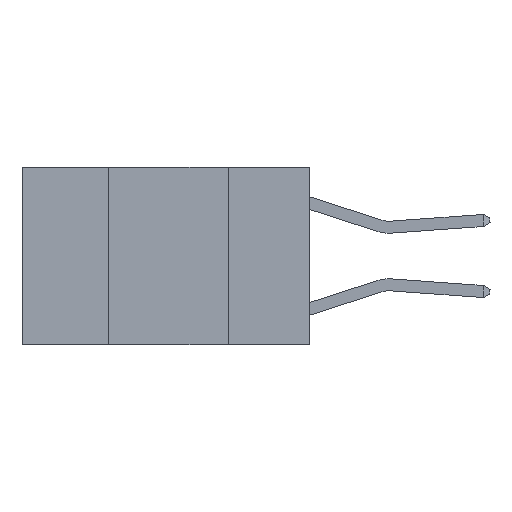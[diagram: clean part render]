
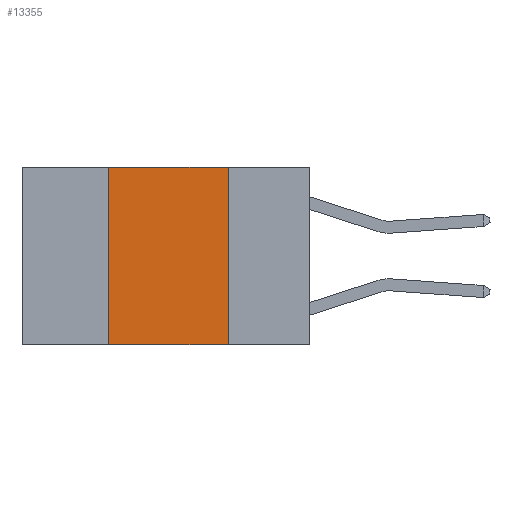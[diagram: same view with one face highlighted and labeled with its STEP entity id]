
A CAD part, left-side view. The second image highlights one B-rep face of the part: STEP entity #13355.
In plain terms, the highlighted planar face has unit normal (-1, 0, 0).
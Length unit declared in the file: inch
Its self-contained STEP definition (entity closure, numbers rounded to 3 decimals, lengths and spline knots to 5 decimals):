
#691 = DIRECTION ( 'NONE',  ( 1., 0., 0. ) ) ;
#2619 = VERTEX_POINT ( 'NONE', #2641 ) ;
#2641 = CARTESIAN_POINT ( 'NONE',  ( 0., 0.42, -0.37 ) ) ;
#3017 = CARTESIAN_POINT ( 'NONE',  ( 0., 0.6, 0. ) ) ;
#3070 = VERTEX_POINT ( 'NONE', #6772 ) ;
#3686 = ORIENTED_EDGE ( 'NONE', *, *, #6469, .F. ) ;
#4028 = DIRECTION ( 'NONE',  ( 0., 0., 1. ) ) ;
#4128 = LINE ( 'NONE', #18617, #9980 ) ;
#4598 = EDGE_LOOP ( 'NONE', ( #11646, #3686, #17595, #8081 ) ) ;
#5270 = CARTESIAN_POINT ( 'NONE',  ( 0., 0.42, 0. ) ) ;
#5556 = DIRECTION ( 'NONE',  ( 0., -1., 0. ) ) ;
#6261 = DIRECTION ( 'NONE',  ( 0., -1., 0. ) ) ;
#6469 = EDGE_CURVE ( 'NONE', #12246, #11231, #10137, .T. ) ;
#6736 = CARTESIAN_POINT ( 'NONE',  ( 0., 0.17, 0. ) ) ;
#6772 = CARTESIAN_POINT ( 'NONE',  ( 0., 0.17, -0.37 ) ) ;
#7762 = CARTESIAN_POINT ( 'NONE',  ( 0., 0.42, 0. ) ) ;
#8081 = ORIENTED_EDGE ( 'NONE', *, *, #17845, .T. ) ;
#8276 = AXIS2_PLACEMENT_3D ( 'NONE', #16616, #691, #12301 ) ;
#9980 = VECTOR ( 'NONE', #5556, 39.37008 ) ;
#10137 = LINE ( 'NONE', #3017, #11851 ) ;
#10649 = EDGE_CURVE ( 'NONE', #2619, #12246, #17094, .T. ) ;
#10750 = FACE_OUTER_BOUND ( 'NONE', #4598, .T. ) ;
#11231 = VERTEX_POINT ( 'NONE', #14378 ) ;
#11646 = ORIENTED_EDGE ( 'NONE', *, *, #16770, .F. ) ;
#11851 = VECTOR ( 'NONE', #6261, 39.37008 ) ;
#12246 = VERTEX_POINT ( 'NONE', #7762 ) ;
#12301 = DIRECTION ( 'NONE',  ( 0., 0., -1. ) ) ;
#12533 = DIRECTION ( 'NONE',  ( 0., 0., -1. ) ) ;
#13355 = ADVANCED_FACE ( 'NONE', ( #10750 ), #15178, .F. ) ;
#14378 = CARTESIAN_POINT ( 'NONE',  ( 0., 0.17, 0. ) ) ;
#15178 = PLANE ( 'NONE',  #8276 ) ;
#16616 = CARTESIAN_POINT ( 'NONE',  ( 0., 0.6, 0. ) ) ;
#16770 = EDGE_CURVE ( 'NONE', #11231, #3070, #18306, .T. ) ;
#17094 = LINE ( 'NONE', #5270, #17450 ) ;
#17300 = VECTOR ( 'NONE', #12533, 39.37008 ) ;
#17450 = VECTOR ( 'NONE', #4028, 39.37008 ) ;
#17595 = ORIENTED_EDGE ( 'NONE', *, *, #10649, .F. ) ;
#17845 = EDGE_CURVE ( 'NONE', #2619, #3070, #4128, .T. ) ;
#18306 = LINE ( 'NONE', #6736, #17300 ) ;
#18617 = CARTESIAN_POINT ( 'NONE',  ( 0., 0.6, -0.37 ) ) ;
